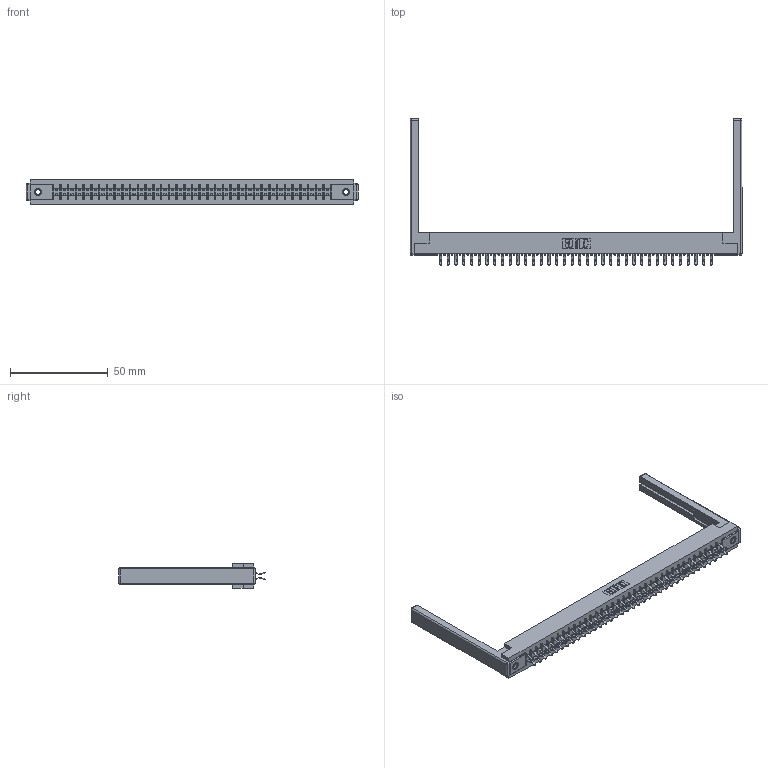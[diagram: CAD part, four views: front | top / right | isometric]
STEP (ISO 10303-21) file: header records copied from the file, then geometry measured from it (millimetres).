
FILE_DESCRIPTION (( 'STEP AP203' ), '1' );
FILE_NAME ('315-072-556-268.STEP', '2019-09-10T21:57:48', ( '' ), ( '' ), 'SwSTEP 2.0', 'SolidWorks 2016', '' );
FILE_SCHEMA (( 'CONFIG_CONTROL_DESIGN' ));
Length unit declared in the file: inch
Products named in the file (5): 315-072-556-268; 305 Part_.156 Dia; 307-220-068; 305-290-001_556; 345-250-001_345-250-001-102
Assembly tree (77 placements, depth 2):
  315-072-556-268
    305 Part_.156 Dia
    305-290-001_556  x72
    345-250-001_345-250-001-102  x2
    307-220-068  x2
Bounding box: 170.08 x 74.93 x 12.7 mm (x, y, z)
Volume: 22088.3 mm3; surface area: 26367.5 mm2
Topology: 77 solids, 77 shells, 4302 faces, 12334 edges, 8008 vertices
Faces by surface type: plane 2388, cylinder 1746, sphere 152, cone 12, torus 4
Entity records: 42690 total; most frequent: CARTESIAN_POINT 7039, ORIENTED_EDGE 6978, DIRECTION 6837, EDGE_CURVE 3489, VECTOR 2801, LINE 2801, VERTEX_POINT 2220, AXIS2_PLACEMENT_3D 2018
